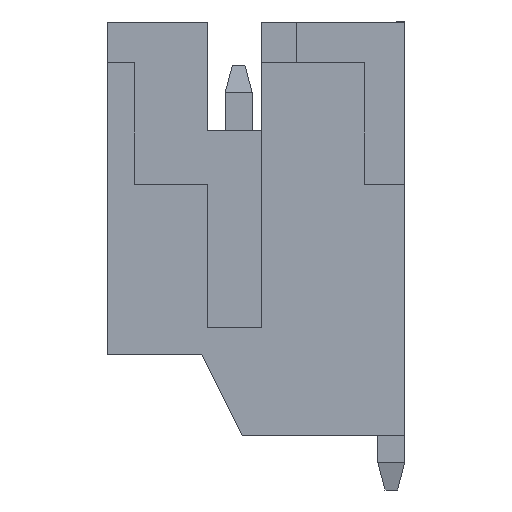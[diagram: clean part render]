
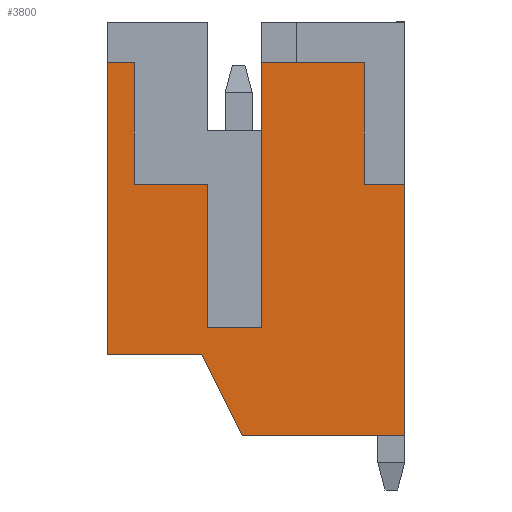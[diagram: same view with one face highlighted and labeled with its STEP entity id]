
A CAD part, left-side view. The second image highlights one B-rep face of the part: STEP entity #3800.
In plain terms, the highlighted planar face has unit normal (-1, 0, 0).
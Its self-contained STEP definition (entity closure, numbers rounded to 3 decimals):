
#45 = EDGE_CURVE ( 'NONE', #1174, #9172, #8184, .T. ) ;
#54 = CARTESIAN_POINT ( 'NONE',  ( -3., 0.68, 0. ) ) ;
#149 = CARTESIAN_POINT ( 'NONE',  ( -3., 0.58, 3.15 ) ) ;
#167 = ORIENTED_EDGE ( 'NONE', *, *, #45, .T. ) ;
#474 = VECTOR ( 'NONE', #4051, 1000. ) ;
#635 = CARTESIAN_POINT ( 'NONE',  ( -3., 2.43, 0. ) ) ;
#851 = LINE ( 'NONE', #8890, #2947 ) ;
#872 = DIRECTION ( 'NONE',  ( 0., 0., 1. ) ) ;
#948 = VECTOR ( 'NONE', #6235, 1000. ) ;
#1147 = EDGE_CURVE ( 'NONE', #1511, #9321, #9761, .T. ) ;
#1174 = VERTEX_POINT ( 'NONE', #3533 ) ;
#1292 = ORIENTED_EDGE ( 'NONE', *, *, #8020, .F. ) ;
#1405 = VECTOR ( 'NONE', #4057, 1000. ) ;
#1511 = VERTEX_POINT ( 'NONE', #2278 ) ;
#1574 = VERTEX_POINT ( 'NONE', #6507 ) ;
#1733 = EDGE_CURVE ( 'NONE', #8605, #6091, #1788, .T. ) ;
#1788 = LINE ( 'NONE', #5865, #5818 ) ;
#1798 = ORIENTED_EDGE ( 'NONE', *, *, #3985, .F. ) ;
#1810 = CARTESIAN_POINT ( 'NONE',  ( -3., 2.43, 0. ) ) ;
#1981 = FACE_OUTER_BOUND ( 'NONE', #7413, .T. ) ;
#2005 = VECTOR ( 'NONE', #2710, 1000. ) ;
#2083 = VECTOR ( 'NONE', #7700, 1000. ) ;
#2275 = CARTESIAN_POINT ( 'NONE',  ( -3., 1.93, 3.15 ) ) ;
#2278 = CARTESIAN_POINT ( 'NONE',  ( -3., -2.32, 3.15 ) ) ;
#2321 = VECTOR ( 'NONE', #3107, 1000. ) ;
#2400 = CARTESIAN_POINT ( 'NONE',  ( -3., -0.42, 5.4 ) ) ;
#2460 = ORIENTED_EDGE ( 'NONE', *, *, #3160, .T. ) ;
#2543 = CARTESIAN_POINT ( 'NONE',  ( -3., -3.07, -1.5 ) ) ;
#2605 = EDGE_CURVE ( 'NONE', #7165, #1574, #6656, .T. ) ;
#2710 = DIRECTION ( 'NONE',  ( 0., 0., 1. ) ) ;
#2714 = CARTESIAN_POINT ( 'NONE',  ( -3., -2.32, 3.15 ) ) ;
#2745 = DIRECTION ( 'NONE',  ( 0., 0., -1. ) ) ;
#2826 = AXIS2_PLACEMENT_3D ( 'NONE', #8222, #3610, #4392 ) ;
#2852 = PLANE ( 'NONE',  #2826 ) ;
#2946 = VERTEX_POINT ( 'NONE', #635 ) ;
#2947 = VECTOR ( 'NONE', #6658, 1000. ) ;
#3107 = DIRECTION ( 'NONE',  ( 0., 0., -1. ) ) ;
#3160 = EDGE_CURVE ( 'NONE', #8460, #1174, #6518, .T. ) ;
#3178 = CARTESIAN_POINT ( 'NONE',  ( -3., 0.58, 3.15 ) ) ;
#3383 = EDGE_CURVE ( 'NONE', #2946, #8460, #3393, .T. ) ;
#3393 = LINE ( 'NONE', #1810, #474 ) ;
#3457 = CARTESIAN_POINT ( 'NONE',  ( -3., 0.58, 0.5 ) ) ;
#3476 = LINE ( 'NONE', #8804, #8635 ) ;
#3533 = CARTESIAN_POINT ( 'NONE',  ( -3., -0.07, -1.5 ) ) ;
#3610 = DIRECTION ( 'NONE',  ( -1., 0., 0. ) ) ;
#3624 = CARTESIAN_POINT ( 'NONE',  ( -3., -0.42, 6.15 ) ) ;
#3800 = ADVANCED_FACE ( 'NONE', ( #1981 ), #2852, .T. ) ;
#3831 = CARTESIAN_POINT ( 'NONE',  ( -3., -3.07, -1.5 ) ) ;
#3944 = ORIENTED_EDGE ( 'NONE', *, *, #7886, .T. ) ;
#3985 = EDGE_CURVE ( 'NONE', #5398, #6845, #6745, .T. ) ;
#4051 = DIRECTION ( 'NONE',  ( 0., -1., 0. ) ) ;
#4057 = DIRECTION ( 'NONE',  ( 0., -1., 0. ) ) ;
#4159 = DIRECTION ( 'NONE',  ( 0., 1., 0. ) ) ;
#4253 = CARTESIAN_POINT ( 'NONE',  ( -3., -2.32, 3.15 ) ) ;
#4373 = CARTESIAN_POINT ( 'NONE',  ( -3., 2.43, 5.4 ) ) ;
#4392 = DIRECTION ( 'NONE',  ( 0., -1., 0. ) ) ;
#4536 = ORIENTED_EDGE ( 'NONE', *, *, #9778, .F. ) ;
#4548 = EDGE_CURVE ( 'NONE', #5850, #2946, #7578, .T. ) ;
#4868 = ORIENTED_EDGE ( 'NONE', *, *, #3383, .T. ) ;
#4985 = ORIENTED_EDGE ( 'NONE', *, *, #1733, .T. ) ;
#4988 = LINE ( 'NONE', #8724, #2005 ) ;
#5109 = VECTOR ( 'NONE', #6589, 1000. ) ;
#5197 = EDGE_CURVE ( 'NONE', #1574, #5850, #3476, .T. ) ;
#5217 = VECTOR ( 'NONE', #8160, 1000. ) ;
#5398 = VERTEX_POINT ( 'NONE', #149 ) ;
#5543 = LINE ( 'NONE', #7176, #1405 ) ;
#5594 = VECTOR ( 'NONE', #9665, 1000. ) ;
#5633 = ORIENTED_EDGE ( 'NONE', *, *, #4548, .T. ) ;
#5818 = VECTOR ( 'NONE', #5829, 1000. ) ;
#5829 = DIRECTION ( 'NONE',  ( 0., 1., 0. ) ) ;
#5831 = ORIENTED_EDGE ( 'NONE', *, *, #5197, .T. ) ;
#5850 = VERTEX_POINT ( 'NONE', #4373 ) ;
#5865 = CARTESIAN_POINT ( 'NONE',  ( -3., -3.07, 5.4 ) ) ;
#6057 = VECTOR ( 'NONE', #872, 1000. ) ;
#6091 = VERTEX_POINT ( 'NONE', #2400 ) ;
#6151 = CARTESIAN_POINT ( 'NONE',  ( -3., -2.32, 5.4 ) ) ;
#6235 = DIRECTION ( 'NONE',  ( 0., -0.447, -0.894 ) ) ;
#6332 = CARTESIAN_POINT ( 'NONE',  ( -3., 1.93, 3.15 ) ) ;
#6415 = LINE ( 'NONE', #3624, #5217 ) ;
#6480 = CARTESIAN_POINT ( 'NONE',  ( -3., 2.43, 6.15 ) ) ;
#6507 = CARTESIAN_POINT ( 'NONE',  ( -3., 1.93, 5.4 ) ) ;
#6518 = LINE ( 'NONE', #7764, #948 ) ;
#6589 = DIRECTION ( 'NONE',  ( 0., 0., 1. ) ) ;
#6656 = LINE ( 'NONE', #2275, #6057 ) ;
#6658 = DIRECTION ( 'NONE',  ( 0., -1., 0. ) ) ;
#6681 = CARTESIAN_POINT ( 'NONE',  ( -3., -3.07, 3.15 ) ) ;
#6745 = LINE ( 'NONE', #3178, #2321 ) ;
#6845 = VERTEX_POINT ( 'NONE', #3457 ) ;
#7028 = LINE ( 'NONE', #4253, #5109 ) ;
#7165 = VERTEX_POINT ( 'NONE', #6332 ) ;
#7176 = CARTESIAN_POINT ( 'NONE',  ( -3., -0.42, 0.5 ) ) ;
#7413 = EDGE_LOOP ( 'NONE', ( #5831, #5633, #4868, #2460, #167, #9584, #7690, #8603, #4985, #3944, #4536, #1798, #1292, #8881 ) ) ;
#7469 = EDGE_CURVE ( 'NONE', #1511, #8605, #7028, .T. ) ;
#7578 = LINE ( 'NONE', #6480, #9348 ) ;
#7690 = ORIENTED_EDGE ( 'NONE', *, *, #1147, .F. ) ;
#7700 = DIRECTION ( 'NONE',  ( 0., -1., 0. ) ) ;
#7764 = CARTESIAN_POINT ( 'NONE',  ( -3., -0.07, -1.5 ) ) ;
#7886 = EDGE_CURVE ( 'NONE', #6091, #8404, #6415, .T. ) ;
#8020 = EDGE_CURVE ( 'NONE', #7165, #5398, #851, .T. ) ;
#8160 = DIRECTION ( 'NONE',  ( 0., 0., -1. ) ) ;
#8184 = LINE ( 'NONE', #3831, #2083 ) ;
#8222 = CARTESIAN_POINT ( 'NONE',  ( -3., 0., 0. ) ) ;
#8384 = EDGE_CURVE ( 'NONE', #9172, #9321, #4988, .T. ) ;
#8404 = VERTEX_POINT ( 'NONE', #8821 ) ;
#8460 = VERTEX_POINT ( 'NONE', #54 ) ;
#8603 = ORIENTED_EDGE ( 'NONE', *, *, #7469, .T. ) ;
#8605 = VERTEX_POINT ( 'NONE', #6151 ) ;
#8635 = VECTOR ( 'NONE', #4159, 1000. ) ;
#8724 = CARTESIAN_POINT ( 'NONE',  ( -3., -3.07, 6.15 ) ) ;
#8804 = CARTESIAN_POINT ( 'NONE',  ( -3., -3.07, 5.4 ) ) ;
#8821 = CARTESIAN_POINT ( 'NONE',  ( -3., -0.42, 0.5 ) ) ;
#8881 = ORIENTED_EDGE ( 'NONE', *, *, #2605, .T. ) ;
#8890 = CARTESIAN_POINT ( 'NONE',  ( -3., -0.42, 3.15 ) ) ;
#9172 = VERTEX_POINT ( 'NONE', #2543 ) ;
#9321 = VERTEX_POINT ( 'NONE', #6681 ) ;
#9348 = VECTOR ( 'NONE', #2745, 1000. ) ;
#9584 = ORIENTED_EDGE ( 'NONE', *, *, #8384, .T. ) ;
#9665 = DIRECTION ( 'NONE',  ( 0., -1., 0. ) ) ;
#9761 = LINE ( 'NONE', #2714, #5594 ) ;
#9778 = EDGE_CURVE ( 'NONE', #6845, #8404, #5543, .T. ) ;
